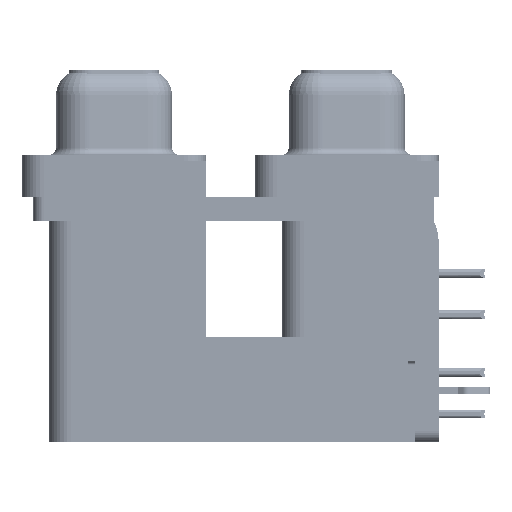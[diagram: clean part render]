
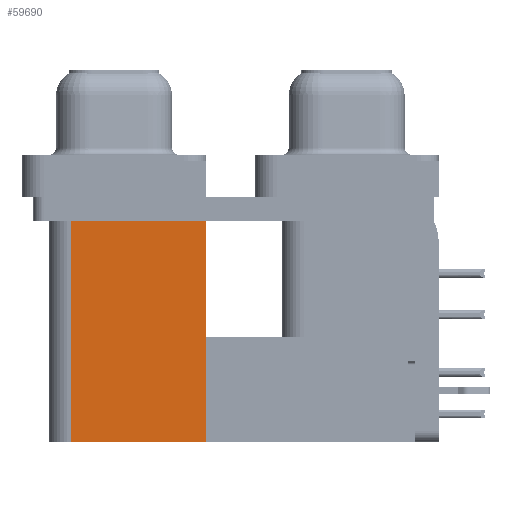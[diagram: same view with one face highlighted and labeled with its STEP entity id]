
A CAD part, left-side view. The second image highlights one B-rep face of the part: STEP entity #59690.
In plain terms, the highlighted planar face has unit normal (-1, 0, 0).
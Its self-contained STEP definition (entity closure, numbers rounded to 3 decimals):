
#403 = DIRECTION ( 'NONE',  ( 1., 0., 0. ) ) ;
#1154 = PLANE ( 'NONE',  #49916 ) ;
#2049 = EDGE_CURVE ( 'NONE', #25769, #68474, #12425, .T. ) ;
#5144 = EDGE_CURVE ( 'NONE', #25880, #61907, #40161, .T. ) ;
#6813 = ORIENTED_EDGE ( 'NONE', *, *, #15113, .T. ) ;
#9954 = ORIENTED_EDGE ( 'NONE', *, *, #2049, .T. ) ;
#11143 = DIRECTION ( 'NONE',  ( 0., 1., 0. ) ) ;
#11998 = DIRECTION ( 'NONE',  ( 0., 0., -1. ) ) ;
#12425 = LINE ( 'NONE', #30564, #64101 ) ;
#12736 = FACE_OUTER_BOUND ( 'NONE', #16125, .T. ) ;
#15113 = EDGE_CURVE ( 'NONE', #68474, #61907, #47267, .T. ) ;
#15867 = VECTOR ( 'NONE', #35506, 1000. ) ;
#16125 = EDGE_LOOP ( 'NONE', ( #6813, #40852, #16525, #9954 ) ) ;
#16525 = ORIENTED_EDGE ( 'NONE', *, *, #19490, .F. ) ;
#18690 = CARTESIAN_POINT ( 'NONE',  ( 3.79, 9.6, -2.5 ) ) ;
#19490 = EDGE_CURVE ( 'NONE', #25769, #25880, #58970, .T. ) ;
#21854 = CARTESIAN_POINT ( 'NONE',  ( 3.79, 18.8, -2.5 ) ) ;
#25769 = VERTEX_POINT ( 'NONE', #67693 ) ;
#25880 = VERTEX_POINT ( 'NONE', #74273 ) ;
#28951 = CARTESIAN_POINT ( 'NONE',  ( 3.79, 18.8, -19.2 ) ) ;
#30564 = CARTESIAN_POINT ( 'NONE',  ( 3.79, 9.6, -19.2 ) ) ;
#35506 = DIRECTION ( 'NONE',  ( 0., 0., 1. ) ) ;
#40161 = LINE ( 'NONE', #28951, #15867 ) ;
#40789 = VECTOR ( 'NONE', #64603, 1000. ) ;
#40852 = ORIENTED_EDGE ( 'NONE', *, *, #5144, .F. ) ;
#43623 = CARTESIAN_POINT ( 'NONE',  ( 3.79, 9.6, -2.5 ) ) ;
#47267 = LINE ( 'NONE', #18690, #40789 ) ;
#49916 = AXIS2_PLACEMENT_3D ( 'NONE', #64839, #403, #11998 ) ;
#53520 = VECTOR ( 'NONE', #11143, 1000. ) ;
#58970 = LINE ( 'NONE', #70547, #53520 ) ;
#59690 = ADVANCED_FACE ( 'NONE', ( #12736 ), #1154, .F. ) ;
#61907 = VERTEX_POINT ( 'NONE', #21854 ) ;
#64101 = VECTOR ( 'NONE', #72220, 1000. ) ;
#64603 = DIRECTION ( 'NONE',  ( 0., 1., 0. ) ) ;
#64839 = CARTESIAN_POINT ( 'NONE',  ( 3.79, 9.6, -19.2 ) ) ;
#67693 = CARTESIAN_POINT ( 'NONE',  ( 3.79, 9.6, -19.2 ) ) ;
#68474 = VERTEX_POINT ( 'NONE', #43623 ) ;
#70547 = CARTESIAN_POINT ( 'NONE',  ( 3.79, 9.6, -19.2 ) ) ;
#72220 = DIRECTION ( 'NONE',  ( 0., 0., 1. ) ) ;
#74273 = CARTESIAN_POINT ( 'NONE',  ( 3.79, 18.8, -19.2 ) ) ;
